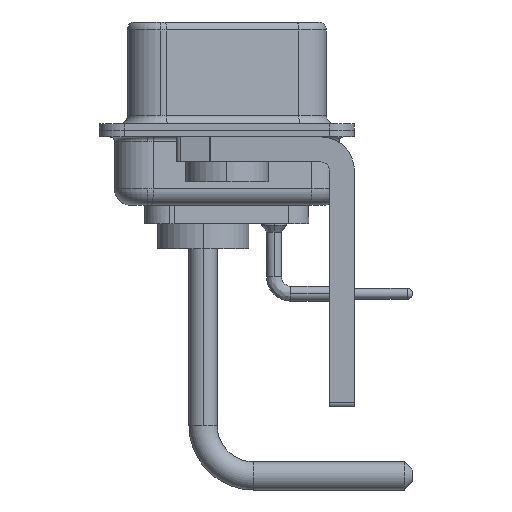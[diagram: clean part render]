
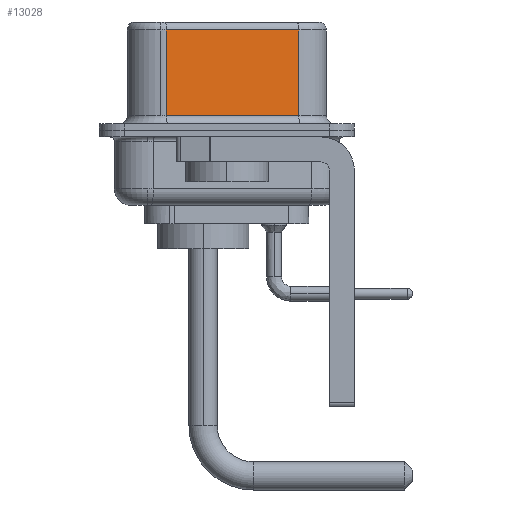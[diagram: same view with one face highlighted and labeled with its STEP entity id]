
A CAD part, left-side view. The second image highlights one B-rep face of the part: STEP entity #13028.
In plain terms, the highlighted planar face has unit normal (-0.985, -0.174, 0).
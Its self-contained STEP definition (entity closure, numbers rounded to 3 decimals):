
#52 = CARTESIAN_POINT ( 'NONE',  ( 3.73, 3.628, 6.52 ) ) ;
#542 = DIRECTION ( 'NONE',  ( 0.174, -0.985, 0. ) ) ;
#2566 = EDGE_LOOP ( 'NONE', ( #9343, #21424, #19517, #15727 ) ) ;
#2743 = VECTOR ( 'NONE', #5761, 1000. ) ;
#3154 = VERTEX_POINT ( 'NONE', #8876 ) ;
#4080 = EDGE_CURVE ( 'NONE', #4732, #23769, #9601, .T. ) ;
#4564 = EDGE_CURVE ( 'NONE', #9526, #23769, #16077, .T. ) ;
#4732 = VERTEX_POINT ( 'NONE', #22556 ) ;
#4940 = CARTESIAN_POINT ( 'NONE',  ( 5.132, -4.322, 0.9 ) ) ;
#5761 = DIRECTION ( 'NONE',  ( -0.174, 0.985, 0. ) ) ;
#6165 = DIRECTION ( 'NONE',  ( -0.174, 0.985, 0. ) ) ;
#6755 = VECTOR ( 'NONE', #542, 1000. ) ;
#7629 = CARTESIAN_POINT ( 'NONE',  ( 5.132, -4.322, 6.02 ) ) ;
#7919 = PLANE ( 'NONE',  #20306 ) ;
#8093 = VECTOR ( 'NONE', #23617, 1000. ) ;
#8413 = CARTESIAN_POINT ( 'NONE',  ( 5.132, -4.322, 6.52 ) ) ;
#8876 = CARTESIAN_POINT ( 'NONE',  ( 3.73, 3.628, 6.02 ) ) ;
#9251 = EDGE_CURVE ( 'NONE', #3154, #4732, #20645, .T. ) ;
#9343 = ORIENTED_EDGE ( 'NONE', *, *, #4564, .F. ) ;
#9526 = VERTEX_POINT ( 'NONE', #20118 ) ;
#9601 = LINE ( 'NONE', #10094, #6755 ) ;
#10094 = CARTESIAN_POINT ( 'NONE',  ( 5.132, -4.322, 0.9 ) ) ;
#13028 = ADVANCED_FACE ( 'NONE', ( #15947 ), #7919, .F. ) ;
#14332 = CARTESIAN_POINT ( 'NONE',  ( 5.132, -4.322, 6.52 ) ) ;
#14520 = EDGE_CURVE ( 'NONE', #9526, #3154, #19051, .T. ) ;
#15699 = DIRECTION ( 'NONE',  ( 0.985, 0.174, 0. ) ) ;
#15727 = ORIENTED_EDGE ( 'NONE', *, *, #4080, .T. ) ;
#15947 = FACE_OUTER_BOUND ( 'NONE', #2566, .T. ) ;
#16077 = LINE ( 'NONE', #14332, #8093 ) ;
#19051 = LINE ( 'NONE', #7629, #2743 ) ;
#19271 = DIRECTION ( 'NONE',  ( 0., 0., -1. ) ) ;
#19517 = ORIENTED_EDGE ( 'NONE', *, *, #9251, .T. ) ;
#20118 = CARTESIAN_POINT ( 'NONE',  ( 5.132, -4.322, 6.02 ) ) ;
#20306 = AXIS2_PLACEMENT_3D ( 'NONE', #8413, #15699, #6165 ) ;
#20645 = LINE ( 'NONE', #52, #24221 ) ;
#21424 = ORIENTED_EDGE ( 'NONE', *, *, #14520, .T. ) ;
#22556 = CARTESIAN_POINT ( 'NONE',  ( 3.73, 3.628, 0.9 ) ) ;
#23617 = DIRECTION ( 'NONE',  ( 0., 0., -1. ) ) ;
#23769 = VERTEX_POINT ( 'NONE', #4940 ) ;
#24221 = VECTOR ( 'NONE', #19271, 1000. ) ;
